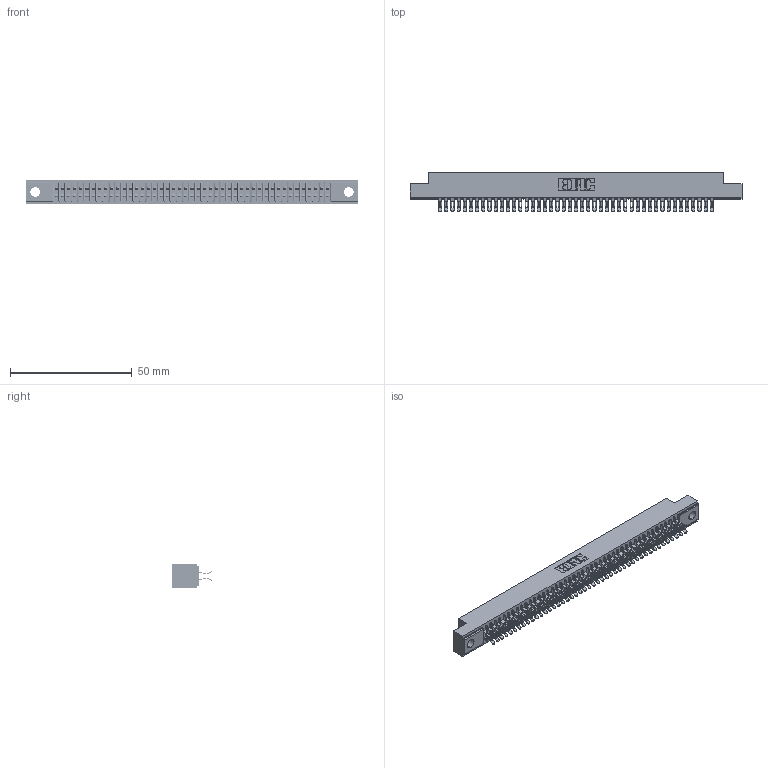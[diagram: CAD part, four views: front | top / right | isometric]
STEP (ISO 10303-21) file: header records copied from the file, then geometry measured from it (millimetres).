
FILE_DESCRIPTION (( 'STEP AP203' ), '1' );
FILE_NAME ('341-090-555-204.STEP', '2018-08-08T00:13:52', ( '' ), ( '' ), 'SwSTEP 2.0', 'SolidWorks 2016', '' );
FILE_SCHEMA (( 'CONFIG_CONTROL_DESIGN' ));
Length unit declared in the file: inch
Products named in the file (3): 341 Part_.156 (3.96) Dia Mounting Holes; 341-292-001_341-292-155; 341-090-555-204
Assembly tree (91 placements, depth 2):
  341-090-555-204
    341 Part_.156 (3.96) Dia Mounting Holes
    341-292-001_341-292-155  x90
Bounding box: 136.53 x 16.31 x 10.16 mm (x, y, z)
Volume: 10092.8 mm3; surface area: 18631.6 mm2
Topology: 91 solids, 91 shells, 7150 faces, 21367 edges, 13910 vertices
Faces by surface type: plane 3862, cylinder 3108, sphere 92, torus 88
Entity records: 54948 total; most frequent: CARTESIAN_POINT 9155, ORIENTED_EDGE 9086, DIRECTION 8865, EDGE_CURVE 4543, VECTOR 3665, LINE 3665, VERTEX_POINT 2874, AXIS2_PLACEMENT_3D 2600
